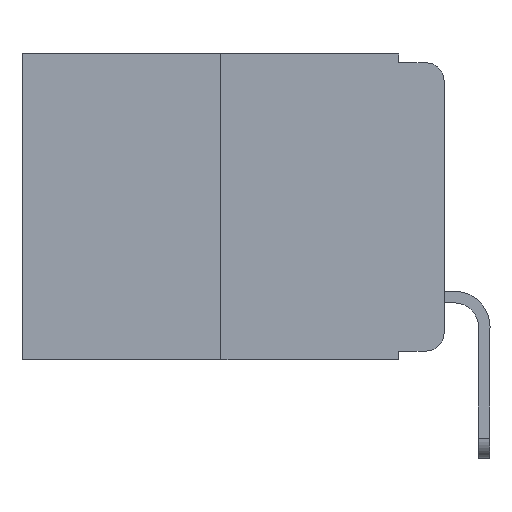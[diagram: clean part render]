
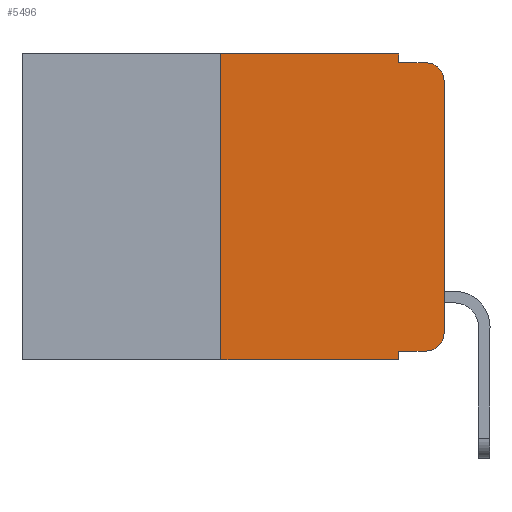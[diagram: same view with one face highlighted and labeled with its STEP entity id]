
A CAD part, left-side view. The second image highlights one B-rep face of the part: STEP entity #5496.
In plain terms, the highlighted planar face has unit normal (-1, 0, 0).
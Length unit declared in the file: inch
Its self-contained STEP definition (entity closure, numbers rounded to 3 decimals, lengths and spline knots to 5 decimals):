
#489 = DIRECTION ( 'NONE',  ( 0., -1., 0. ) ) ;
#783 = EDGE_CURVE ( 'NONE', #16893, #4027, #12003, .T. ) ;
#1021 = CARTESIAN_POINT ( 'NONE',  ( 0., 0.051, 0. ) ) ;
#1026 = VERTEX_POINT ( 'NONE', #16110 ) ;
#1031 = ORIENTED_EDGE ( 'NONE', *, *, #11381, .T. ) ;
#1154 = ORIENTED_EDGE ( 'NONE', *, *, #16476, .F. ) ;
#1334 = EDGE_LOOP ( 'NONE', ( #2208, #1699, #12682, #1154, #1979, #4584, #3585, #3090, #1031, #18161 ) ) ;
#1555 = DIRECTION ( 'NONE',  ( 0., 0., -1. ) ) ;
#1699 = ORIENTED_EDGE ( 'NONE', *, *, #20417, .T. ) ;
#1979 = ORIENTED_EDGE ( 'NONE', *, *, #783, .F. ) ;
#2056 = LINE ( 'NONE', #16113, #10843 ) ;
#2208 = ORIENTED_EDGE ( 'NONE', *, *, #5329, .T. ) ;
#3090 = ORIENTED_EDGE ( 'NONE', *, *, #12437, .F. ) ;
#3248 = VERTEX_POINT ( 'NONE', #12920 ) ;
#3402 = CARTESIAN_POINT ( 'NONE',  ( 0., 0.051, -0.01 ) ) ;
#3563 = VECTOR ( 'NONE', #15023, 39.37008 ) ;
#3585 = ORIENTED_EDGE ( 'NONE', *, *, #19339, .T. ) ;
#3917 = CIRCLE ( 'NONE', #17915, 0.02 ) ;
#4027 = VERTEX_POINT ( 'NONE', #1021 ) ;
#4194 = VECTOR ( 'NONE', #1555, 39.37008 ) ;
#4584 = ORIENTED_EDGE ( 'NONE', *, *, #15490, .F. ) ;
#4753 = CARTESIAN_POINT ( 'NONE',  ( 0., 0.25, 0. ) ) ;
#4993 = CARTESIAN_POINT ( 'NONE',  ( 0., 0., -0.03 ) ) ;
#5148 = LINE ( 'NONE', #18637, #9700 ) ;
#5157 = DIRECTION ( 'NONE',  ( -1., 0., 0. ) ) ;
#5329 = EDGE_CURVE ( 'NONE', #20804, #8665, #11879, .T. ) ;
#5496 = ADVANCED_FACE ( 'NONE', ( #13606 ), #17823, .F. ) ;
#5945 = VERTEX_POINT ( 'NONE', #13026 ) ;
#6181 = DIRECTION ( 'NONE',  ( -1., 0., 0. ) ) ;
#6418 = CARTESIAN_POINT ( 'NONE',  ( 0., 0., 0. ) ) ;
#7460 = DIRECTION ( 'NONE',  ( 0., 0., -1. ) ) ;
#7660 = VECTOR ( 'NONE', #20157, 39.37008 ) ;
#8083 = EDGE_CURVE ( 'NONE', #3248, #20804, #20793, .T. ) ;
#8131 = VERTEX_POINT ( 'NONE', #3402 ) ;
#8342 = VERTEX_POINT ( 'NONE', #11080 ) ;
#8571 = DIRECTION ( 'NONE',  ( 1., 0., 0. ) ) ;
#8665 = VERTEX_POINT ( 'NONE', #4993 ) ;
#9350 = LINE ( 'NONE', #20972, #4194 ) ;
#9700 = VECTOR ( 'NONE', #489, 39.37008 ) ;
#9954 = CARTESIAN_POINT ( 'NONE',  ( 0., 0.051, -0.343 ) ) ;
#10710 = DIRECTION ( 'NONE',  ( 0., 0., 1. ) ) ;
#10843 = VECTOR ( 'NONE', #17594, 39.37008 ) ;
#11080 = CARTESIAN_POINT ( 'NONE',  ( 0., 0.02, -0.01 ) ) ;
#11381 = EDGE_CURVE ( 'NONE', #5945, #3248, #5148, .T. ) ;
#11879 = LINE ( 'NONE', #6418, #19405 ) ;
#12003 = LINE ( 'NONE', #20216, #7660 ) ;
#12152 = LINE ( 'NONE', #12332, #12674 ) ;
#12332 = CARTESIAN_POINT ( 'NONE',  ( 0., 0.051, 0. ) ) ;
#12437 = EDGE_CURVE ( 'NONE', #5945, #16300, #12152, .T. ) ;
#12674 = VECTOR ( 'NONE', #7460, 39.37008 ) ;
#12682 = ORIENTED_EDGE ( 'NONE', *, *, #19460, .F. ) ;
#12920 = CARTESIAN_POINT ( 'NONE',  ( 0., 0.02, -0.333 ) ) ;
#13026 = CARTESIAN_POINT ( 'NONE',  ( 0., 0.051, -0.333 ) ) ;
#13520 = CARTESIAN_POINT ( 'NONE',  ( 0., 0.051, -0.01 ) ) ;
#13606 = FACE_OUTER_BOUND ( 'NONE', #1334, .T. ) ;
#13625 = CARTESIAN_POINT ( 'NONE',  ( 0., 0., -0.313 ) ) ;
#13812 = CARTESIAN_POINT ( 'NONE',  ( 0., 0.25, 0. ) ) ;
#14870 = CARTESIAN_POINT ( 'NONE',  ( 0., 0.473, 0. ) ) ;
#14936 = CARTESIAN_POINT ( 'NONE',  ( 0., 0.02, -0.313 ) ) ;
#15023 = DIRECTION ( 'NONE',  ( 0., -1., 0. ) ) ;
#15490 = EDGE_CURVE ( 'NONE', #1026, #16893, #19905, .T. ) ;
#15762 = CARTESIAN_POINT ( 'NONE',  ( 0., 0.02, -0.03 ) ) ;
#15970 = VECTOR ( 'NONE', #10710, 39.37008 ) ;
#16110 = CARTESIAN_POINT ( 'NONE',  ( 0., 0.25, -0.343 ) ) ;
#16113 = CARTESIAN_POINT ( 'NONE',  ( 0., 0.473, -0.343 ) ) ;
#16300 = VERTEX_POINT ( 'NONE', #9954 ) ;
#16419 = DIRECTION ( 'NONE',  ( 0., 0., -1. ) ) ;
#16476 = EDGE_CURVE ( 'NONE', #4027, #8131, #9350, .T. ) ;
#16566 = LINE ( 'NONE', #13520, #3563 ) ;
#16893 = VERTEX_POINT ( 'NONE', #4753 ) ;
#17246 = DIRECTION ( 'NONE',  ( 0., 0., -1. ) ) ;
#17448 = DIRECTION ( 'NONE',  ( 0., 0., 1. ) ) ;
#17594 = DIRECTION ( 'NONE',  ( 0., -1., 0. ) ) ;
#17644 = AXIS2_PLACEMENT_3D ( 'NONE', #14870, #8571, #19334 ) ;
#17823 = PLANE ( 'NONE',  #17644 ) ;
#17915 = AXIS2_PLACEMENT_3D ( 'NONE', #15762, #6181, #17246 ) ;
#18161 = ORIENTED_EDGE ( 'NONE', *, *, #8083, .T. ) ;
#18637 = CARTESIAN_POINT ( 'NONE',  ( 0., 0.051, -0.333 ) ) ;
#19334 = DIRECTION ( 'NONE',  ( 0., 0., -1. ) ) ;
#19339 = EDGE_CURVE ( 'NONE', #1026, #16300, #2056, .T. ) ;
#19405 = VECTOR ( 'NONE', #17448, 39.37008 ) ;
#19460 = EDGE_CURVE ( 'NONE', #8131, #8342, #16566, .T. ) ;
#19905 = LINE ( 'NONE', #13812, #15970 ) ;
#20157 = DIRECTION ( 'NONE',  ( 0., -1., 0. ) ) ;
#20216 = CARTESIAN_POINT ( 'NONE',  ( 0., 0.473, 0. ) ) ;
#20386 = AXIS2_PLACEMENT_3D ( 'NONE', #14936, #5157, #16419 ) ;
#20417 = EDGE_CURVE ( 'NONE', #8665, #8342, #3917, .T. ) ;
#20793 = CIRCLE ( 'NONE', #20386, 0.02 ) ;
#20804 = VERTEX_POINT ( 'NONE', #13625 ) ;
#20972 = CARTESIAN_POINT ( 'NONE',  ( 0., 0.051, 0. ) ) ;
